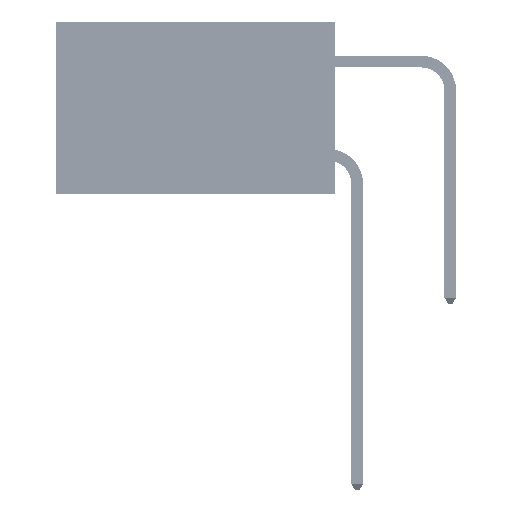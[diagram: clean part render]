
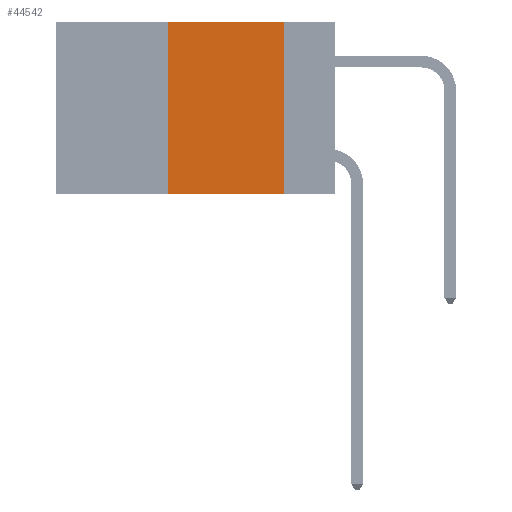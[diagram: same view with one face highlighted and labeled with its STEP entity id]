
A CAD part, left-side view. The second image highlights one B-rep face of the part: STEP entity #44542.
In plain terms, the highlighted planar face has unit normal (-1, 0, 0).
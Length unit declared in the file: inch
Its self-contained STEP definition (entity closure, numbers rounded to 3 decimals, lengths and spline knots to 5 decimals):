
#1049 = ORIENTED_EDGE ( 'NONE', *, *, #45316, .F. ) ;
#2948 = AXIS2_PLACEMENT_3D ( 'NONE', #13187, #12730, #23707 ) ;
#4000 = VERTEX_POINT ( 'NONE', #23677 ) ;
#5341 = VERTEX_POINT ( 'NONE', #20193 ) ;
#6122 = DIRECTION ( 'NONE',  ( 0., 0., -1. ) ) ;
#8698 = LINE ( 'NONE', #23201, #25765 ) ;
#8972 = FACE_OUTER_BOUND ( 'NONE', #24157, .T. ) ;
#9806 = CARTESIAN_POINT ( 'NONE',  ( 0., 0.11, -0.37 ) ) ;
#12730 = DIRECTION ( 'NONE',  ( 1., 0., 0. ) ) ;
#12737 = CARTESIAN_POINT ( 'NONE',  ( 0., 0.36, 0. ) ) ;
#13187 = CARTESIAN_POINT ( 'NONE',  ( 0., 0.6, 0. ) ) ;
#16205 = ORIENTED_EDGE ( 'NONE', *, *, #35521, .F. ) ;
#17462 = VECTOR ( 'NONE', #39818, 39.37008 ) ;
#18361 = EDGE_CURVE ( 'NONE', #5341, #18574, #29489, .T. ) ;
#18574 = VERTEX_POINT ( 'NONE', #9806 ) ;
#20193 = CARTESIAN_POINT ( 'NONE',  ( 0., 0.36, -0.37 ) ) ;
#20902 = LINE ( 'NONE', #12737, #27460 ) ;
#21638 = EDGE_CURVE ( 'NONE', #45455, #18574, #8698, .T. ) ;
#23013 = PLANE ( 'NONE',  #2948 ) ;
#23078 = LINE ( 'NONE', #29186, #36646 ) ;
#23201 = CARTESIAN_POINT ( 'NONE',  ( 0., 0.11, 0. ) ) ;
#23677 = CARTESIAN_POINT ( 'NONE',  ( 0., 0.36, 0. ) ) ;
#23707 = DIRECTION ( 'NONE',  ( 0., 0., -1. ) ) ;
#23952 = DIRECTION ( 'NONE',  ( 0., 0., 1. ) ) ;
#24157 = EDGE_LOOP ( 'NONE', ( #24406, #1049, #16205, #33192 ) ) ;
#24406 = ORIENTED_EDGE ( 'NONE', *, *, #21638, .F. ) ;
#25765 = VECTOR ( 'NONE', #6122, 39.37008 ) ;
#27460 = VECTOR ( 'NONE', #23952, 39.37008 ) ;
#29186 = CARTESIAN_POINT ( 'NONE',  ( 0., 0.6, 0. ) ) ;
#29489 = LINE ( 'NONE', #40514, #17462 ) ;
#32684 = DIRECTION ( 'NONE',  ( 0., -1., 0. ) ) ;
#33192 = ORIENTED_EDGE ( 'NONE', *, *, #18361, .T. ) ;
#34309 = CARTESIAN_POINT ( 'NONE',  ( 0., 0.11, 0. ) ) ;
#35521 = EDGE_CURVE ( 'NONE', #5341, #4000, #20902, .T. ) ;
#36646 = VECTOR ( 'NONE', #32684, 39.37008 ) ;
#39818 = DIRECTION ( 'NONE',  ( 0., -1., 0. ) ) ;
#40514 = CARTESIAN_POINT ( 'NONE',  ( 0., 0.6, -0.37 ) ) ;
#44542 = ADVANCED_FACE ( 'NONE', ( #8972 ), #23013, .F. ) ;
#45316 = EDGE_CURVE ( 'NONE', #4000, #45455, #23078, .T. ) ;
#45455 = VERTEX_POINT ( 'NONE', #34309 ) ;
